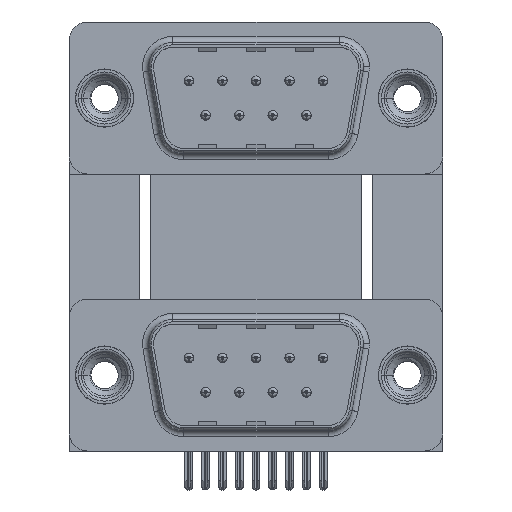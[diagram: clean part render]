
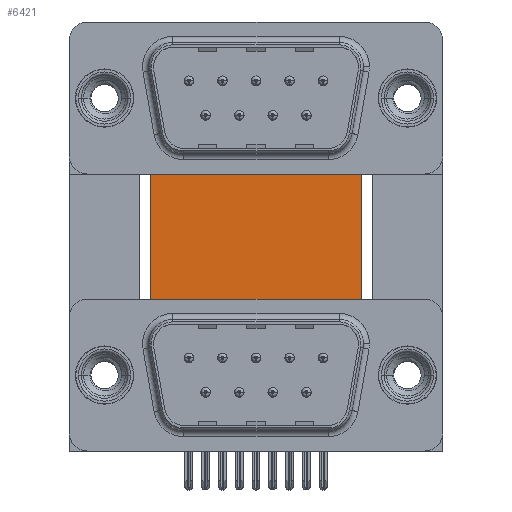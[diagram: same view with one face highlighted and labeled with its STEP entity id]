
A CAD part, top view. The second image highlights one B-rep face of the part: STEP entity #6421.
In plain terms, the highlighted planar face has unit normal (0, 0, 1).
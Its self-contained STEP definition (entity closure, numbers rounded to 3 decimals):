
#131 = EDGE_LOOP ( 'NONE', ( #22860, #7069, #27739, #15156, #208, #13120, #19333, #10571, #20554, #5169 ) ) ;
#152 = CARTESIAN_POINT ( 'NONE',  ( 21.2, 16.585, -12. ) ) ;
#208 = ORIENTED_EDGE ( 'NONE', *, *, #24008, .F. ) ;
#861 = LINE ( 'NONE', #5244, #1926 ) ;
#1088 = DIRECTION ( 'NONE',  ( 1., 0., 0. ) ) ;
#1117 = EDGE_CURVE ( 'NONE', #10923, #6374, #20718, .T. ) ;
#1166 = CARTESIAN_POINT ( 'NONE',  ( 3.79, 16.585, -12. ) ) ;
#1926 = VECTOR ( 'NONE', #9543, 1000. ) ;
#2124 = EDGE_CURVE ( 'NONE', #6374, #24847, #861, .T. ) ;
#2420 = CARTESIAN_POINT ( 'NONE',  ( 22.09, -4.635, -12. ) ) ;
#3299 = FACE_OUTER_BOUND ( 'NONE', #131, .T. ) ;
#3676 = LINE ( 'NONE', #14752, #24340 ) ;
#3850 = VERTEX_POINT ( 'NONE', #21316 ) ;
#3873 = EDGE_CURVE ( 'NONE', #5057, #19687, #12337, .T. ) ;
#3882 = CARTESIAN_POINT ( 'NONE',  ( 21.2, 16.585, -12. ) ) ;
#3938 = CARTESIAN_POINT ( 'NONE',  ( 3.79, -3.735, -12. ) ) ;
#4358 = LINE ( 'NONE', #17032, #14739 ) ;
#5057 = VERTEX_POINT ( 'NONE', #24945 ) ;
#5169 = ORIENTED_EDGE ( 'NONE', *, *, #27871, .T. ) ;
#5244 = CARTESIAN_POINT ( 'NONE',  ( 22.59, -4.635, -12. ) ) ;
#6350 = LINE ( 'NONE', #15166, #14756 ) ;
#6374 = VERTEX_POINT ( 'NONE', #9570 ) ;
#6410 = CARTESIAN_POINT ( 'NONE',  ( 2.9, -4.635, -12. ) ) ;
#6421 = ADVANCED_FACE ( 'NONE', ( #3299 ), #20674, .F. ) ;
#7069 = ORIENTED_EDGE ( 'NONE', *, *, #23090, .T. ) ;
#7766 = VECTOR ( 'NONE', #20991, 1000. ) ;
#7892 = CARTESIAN_POINT ( 'NONE',  ( 21.2, -0.735, -12. ) ) ;
#9079 = AXIS2_PLACEMENT_3D ( 'NONE', #1166, #14536, #18528 ) ;
#9091 = EDGE_CURVE ( 'NONE', #20385, #5057, #6350, .T. ) ;
#9543 = DIRECTION ( 'NONE',  ( -0.336, 0.942, 0. ) ) ;
#9570 = CARTESIAN_POINT ( 'NONE',  ( 22.59, -4.635, -12. ) ) ;
#10020 = DIRECTION ( 'NONE',  ( 0., -1., 0. ) ) ;
#10571 = ORIENTED_EDGE ( 'NONE', *, *, #9091, .T. ) ;
#10923 = VERTEX_POINT ( 'NONE', #2420 ) ;
#10962 = LINE ( 'NONE', #152, #19770 ) ;
#12337 = LINE ( 'NONE', #17891, #25869 ) ;
#13120 = ORIENTED_EDGE ( 'NONE', *, *, #16298, .F. ) ;
#13452 = EDGE_CURVE ( 'NONE', #24431, #27452, #23470, .T. ) ;
#14536 = DIRECTION ( 'NONE',  ( 0., 0., -1. ) ) ;
#14613 = DIRECTION ( 'NONE',  ( 0., 1., 0. ) ) ;
#14739 = VECTOR ( 'NONE', #17320, 1000. ) ;
#14752 = CARTESIAN_POINT ( 'NONE',  ( 2.9, -3.735, -12. ) ) ;
#14756 = VECTOR ( 'NONE', #22042, 1000. ) ;
#14837 = LINE ( 'NONE', #21406, #16737 ) ;
#15156 = ORIENTED_EDGE ( 'NONE', *, *, #2124, .T. ) ;
#15166 = CARTESIAN_POINT ( 'NONE',  ( 2.4, -4.635, -12. ) ) ;
#16298 = EDGE_CURVE ( 'NONE', #3850, #20469, #18701, .T. ) ;
#16737 = VECTOR ( 'NONE', #10020, 1000. ) ;
#17032 = CARTESIAN_POINT ( 'NONE',  ( 3.79, 16.585, -12. ) ) ;
#17320 = DIRECTION ( 'NONE',  ( 0., -1., 0. ) ) ;
#17891 = CARTESIAN_POINT ( 'NONE',  ( 2.9, -4.635, -12. ) ) ;
#18427 = DIRECTION ( 'NONE',  ( 1., 0., 0. ) ) ;
#18528 = DIRECTION ( 'NONE',  ( -1., 0., 0. ) ) ;
#18701 = LINE ( 'NONE', #27713, #27297 ) ;
#18846 = CARTESIAN_POINT ( 'NONE',  ( 22.09, -4.635, -12. ) ) ;
#19049 = EDGE_CURVE ( 'NONE', #3850, #20385, #4358, .T. ) ;
#19333 = ORIENTED_EDGE ( 'NONE', *, *, #19049, .T. ) ;
#19687 = VERTEX_POINT ( 'NONE', #6410 ) ;
#19747 = DIRECTION ( 'NONE',  ( 1., 0., 0. ) ) ;
#19770 = VECTOR ( 'NONE', #27799, 1000. ) ;
#20385 = VERTEX_POINT ( 'NONE', #27828 ) ;
#20469 = VERTEX_POINT ( 'NONE', #3882 ) ;
#20554 = ORIENTED_EDGE ( 'NONE', *, *, #3873, .T. ) ;
#20674 = PLANE ( 'NONE',  #9079 ) ;
#20718 = LINE ( 'NONE', #18846, #7766 ) ;
#20991 = DIRECTION ( 'NONE',  ( 1., 0., 0. ) ) ;
#21316 = CARTESIAN_POINT ( 'NONE',  ( 3.79, 16.585, -12. ) ) ;
#21406 = CARTESIAN_POINT ( 'NONE',  ( 22.09, -3.735, -12. ) ) ;
#21734 = VECTOR ( 'NONE', #1088, 1000. ) ;
#22042 = DIRECTION ( 'NONE',  ( -0.336, -0.942, 0. ) ) ;
#22860 = ORIENTED_EDGE ( 'NONE', *, *, #13452, .T. ) ;
#23090 = EDGE_CURVE ( 'NONE', #27452, #10923, #14837, .T. ) ;
#23470 = LINE ( 'NONE', #3938, #21734 ) ;
#24008 = EDGE_CURVE ( 'NONE', #20469, #24847, #10962, .T. ) ;
#24340 = VECTOR ( 'NONE', #14613, 1000. ) ;
#24431 = VERTEX_POINT ( 'NONE', #27059 ) ;
#24847 = VERTEX_POINT ( 'NONE', #7892 ) ;
#24945 = CARTESIAN_POINT ( 'NONE',  ( 2.4, -4.635, -12. ) ) ;
#25698 = CARTESIAN_POINT ( 'NONE',  ( 22.09, -3.735, -12. ) ) ;
#25869 = VECTOR ( 'NONE', #19747, 1000. ) ;
#27059 = CARTESIAN_POINT ( 'NONE',  ( 2.9, -3.735, -12. ) ) ;
#27297 = VECTOR ( 'NONE', #18427, 1000. ) ;
#27452 = VERTEX_POINT ( 'NONE', #25698 ) ;
#27713 = CARTESIAN_POINT ( 'NONE',  ( 3.79, 16.585, -12. ) ) ;
#27739 = ORIENTED_EDGE ( 'NONE', *, *, #1117, .T. ) ;
#27799 = DIRECTION ( 'NONE',  ( 0., -1., 0. ) ) ;
#27828 = CARTESIAN_POINT ( 'NONE',  ( 3.79, -0.735, -12. ) ) ;
#27871 = EDGE_CURVE ( 'NONE', #19687, #24431, #3676, .T. ) ;
